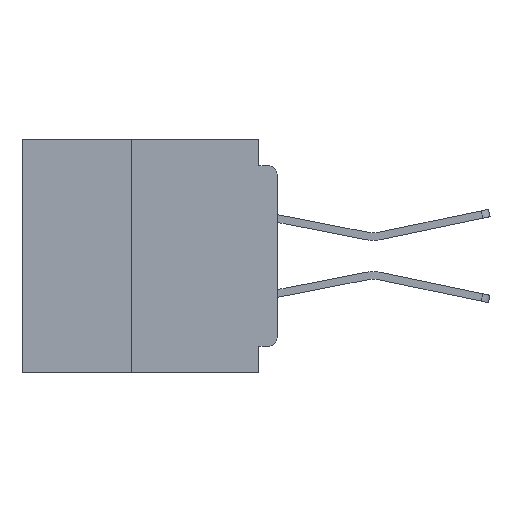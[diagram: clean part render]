
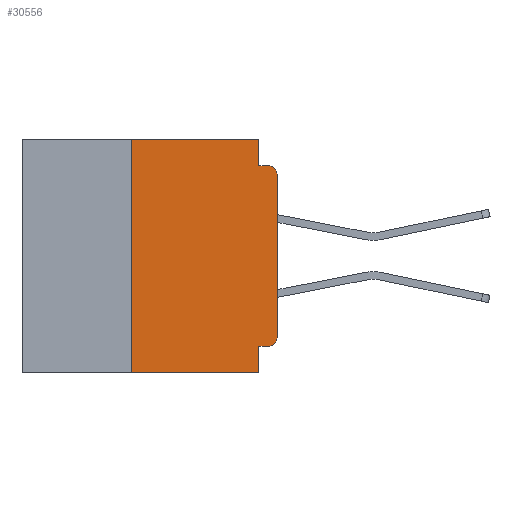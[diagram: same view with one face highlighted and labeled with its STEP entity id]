
A CAD part, left-side view. The second image highlights one B-rep face of the part: STEP entity #30556.
In plain terms, the highlighted planar face has unit normal (-1, 0, 0).
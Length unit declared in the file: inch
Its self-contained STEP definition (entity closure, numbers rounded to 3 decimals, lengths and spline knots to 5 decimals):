
#1017 = VECTOR ( 'NONE', #9681, 39.37008 ) ;
#1236 = VERTEX_POINT ( 'NONE', #1339 ) ;
#1339 = CARTESIAN_POINT ( 'NONE',  ( 0., 0.015, -0.045 ) ) ;
#1862 = ORIENTED_EDGE ( 'NONE', *, *, #42022, .F. ) ;
#1896 = ORIENTED_EDGE ( 'NONE', *, *, #35441, .F. ) ;
#3460 = VECTOR ( 'NONE', #53375, 39.37008 ) ;
#4690 = LINE ( 'NONE', #44997, #47994 ) ;
#5162 = DIRECTION ( 'NONE',  ( 0., -1., 0. ) ) ;
#5245 = VERTEX_POINT ( 'NONE', #38163 ) ;
#5361 = ORIENTED_EDGE ( 'NONE', *, *, #27050, .T. ) ;
#5423 = CARTESIAN_POINT ( 'NONE',  ( 0., 0.437, -0.4 ) ) ;
#6847 = ORIENTED_EDGE ( 'NONE', *, *, #15869, .F. ) ;
#7139 = CARTESIAN_POINT ( 'NONE',  ( 0., 0., 0. ) ) ;
#7909 = VECTOR ( 'NONE', #19508, 39.37008 ) ;
#8006 = DIRECTION ( 'NONE',  ( 1., 0., 0. ) ) ;
#8159 = VERTEX_POINT ( 'NONE', #43054 ) ;
#8168 = CIRCLE ( 'NONE', #32516, 0.015 ) ;
#8342 = ORIENTED_EDGE ( 'NONE', *, *, #15231, .T. ) ;
#9681 = DIRECTION ( 'NONE',  ( 0., -1., 0. ) ) ;
#10176 = AXIS2_PLACEMENT_3D ( 'NONE', #38931, #13913, #43147 ) ;
#11632 = DIRECTION ( 'NONE',  ( 0., -1., 0. ) ) ;
#11812 = CARTESIAN_POINT ( 'NONE',  ( 0., 0.437, 0. ) ) ;
#13487 = CARTESIAN_POINT ( 'NONE',  ( 0., 0.25, -0.4 ) ) ;
#13815 = CARTESIAN_POINT ( 'NONE',  ( 0., 0.031, -0.4 ) ) ;
#13913 = DIRECTION ( 'NONE',  ( -1., 0., 0. ) ) ;
#14528 = CARTESIAN_POINT ( 'NONE',  ( 0., 0.031, 0. ) ) ;
#14894 = VERTEX_POINT ( 'NONE', #17578 ) ;
#15231 = EDGE_CURVE ( 'NONE', #5245, #53070, #37618, .T. ) ;
#15804 = VERTEX_POINT ( 'NONE', #32014 ) ;
#15869 = EDGE_CURVE ( 'NONE', #14894, #30170, #4690, .T. ) ;
#16266 = EDGE_CURVE ( 'NONE', #15804, #14894, #40784, .T. ) ;
#17531 = VERTEX_POINT ( 'NONE', #14528 ) ;
#17578 = CARTESIAN_POINT ( 'NONE',  ( 0., 0.031, -0.355 ) ) ;
#18138 = ORIENTED_EDGE ( 'NONE', *, *, #53557, .T. ) ;
#19508 = DIRECTION ( 'NONE',  ( 0., 0., -1. ) ) ;
#21286 = FACE_OUTER_BOUND ( 'NONE', #34796, .T. ) ;
#22090 = DIRECTION ( 'NONE',  ( -1., 0., 0. ) ) ;
#22170 = VERTEX_POINT ( 'NONE', #13487 ) ;
#23447 = CARTESIAN_POINT ( 'NONE',  ( 0., 0., -0.355 ) ) ;
#23816 = VECTOR ( 'NONE', #11632, 39.37008 ) ;
#25314 = ORIENTED_EDGE ( 'NONE', *, *, #38637, .F. ) ;
#26413 = LINE ( 'NONE', #11812, #23816 ) ;
#27050 = EDGE_CURVE ( 'NONE', #22170, #30170, #34621, .T. ) ;
#28371 = DIRECTION ( 'NONE',  ( 0., 0., -1. ) ) ;
#28968 = PLANE ( 'NONE',  #41947 ) ;
#29868 = EDGE_CURVE ( 'NONE', #22170, #34425, #36995, .T. ) ;
#30170 = VERTEX_POINT ( 'NONE', #13815 ) ;
#30267 = LINE ( 'NONE', #52787, #7909 ) ;
#30556 = ADVANCED_FACE ( 'NONE', ( #21286 ), #28968, .F. ) ;
#31398 = CARTESIAN_POINT ( 'NONE',  ( 0., 0., -0.06 ) ) ;
#32014 = CARTESIAN_POINT ( 'NONE',  ( 0., 0.015, -0.355 ) ) ;
#32516 = AXIS2_PLACEMENT_3D ( 'NONE', #47049, #22090, #51180 ) ;
#32575 = CIRCLE ( 'NONE', #10176, 0.015 ) ;
#32666 = LINE ( 'NONE', #51106, #53475 ) ;
#32994 = ORIENTED_EDGE ( 'NONE', *, *, #29868, .F. ) ;
#34425 = VERTEX_POINT ( 'NONE', #48757 ) ;
#34621 = LINE ( 'NONE', #5423, #1017 ) ;
#34796 = EDGE_LOOP ( 'NONE', ( #8342, #18138, #25314, #1896, #1862, #32994, #5361, #6847, #50646, #39757 ) ) ;
#35441 = EDGE_CURVE ( 'NONE', #17531, #8159, #30267, .T. ) ;
#36465 = DIRECTION ( 'NONE',  ( 0., 0., 1. ) ) ;
#36995 = LINE ( 'NONE', #45095, #3460 ) ;
#37329 = DIRECTION ( 'NONE',  ( 0., 0., -1. ) ) ;
#37618 = LINE ( 'NONE', #7139, #48718 ) ;
#38163 = CARTESIAN_POINT ( 'NONE',  ( 0., 0., -0.34 ) ) ;
#38637 = EDGE_CURVE ( 'NONE', #8159, #1236, #32666, .T. ) ;
#38931 = CARTESIAN_POINT ( 'NONE',  ( 0., 0.015, -0.34 ) ) ;
#39757 = ORIENTED_EDGE ( 'NONE', *, *, #45279, .T. ) ;
#40784 = LINE ( 'NONE', #23447, #53091 ) ;
#41947 = AXIS2_PLACEMENT_3D ( 'NONE', #49707, #8006, #37329 ) ;
#42022 = EDGE_CURVE ( 'NONE', #34425, #17531, #26413, .T. ) ;
#43054 = CARTESIAN_POINT ( 'NONE',  ( 0., 0.031, -0.045 ) ) ;
#43147 = DIRECTION ( 'NONE',  ( 0., 0., -1. ) ) ;
#44997 = CARTESIAN_POINT ( 'NONE',  ( 0., 0.031, -0.4 ) ) ;
#45095 = CARTESIAN_POINT ( 'NONE',  ( 0., 0.25, -0.4 ) ) ;
#45279 = EDGE_CURVE ( 'NONE', #15804, #5245, #32575, .T. ) ;
#47049 = CARTESIAN_POINT ( 'NONE',  ( 0., 0.015, -0.06 ) ) ;
#47994 = VECTOR ( 'NONE', #28371, 39.37008 ) ;
#48718 = VECTOR ( 'NONE', #36465, 39.37008 ) ;
#48757 = CARTESIAN_POINT ( 'NONE',  ( 0., 0.25, 0. ) ) ;
#49707 = CARTESIAN_POINT ( 'NONE',  ( 0., 0.437, 0. ) ) ;
#50646 = ORIENTED_EDGE ( 'NONE', *, *, #16266, .F. ) ;
#51106 = CARTESIAN_POINT ( 'NONE',  ( 0., 0., -0.045 ) ) ;
#51180 = DIRECTION ( 'NONE',  ( 0., 0., -1. ) ) ;
#52533 = DIRECTION ( 'NONE',  ( 0., 1., 0. ) ) ;
#52787 = CARTESIAN_POINT ( 'NONE',  ( 0., 0.031, 0. ) ) ;
#53070 = VERTEX_POINT ( 'NONE', #31398 ) ;
#53091 = VECTOR ( 'NONE', #52533, 39.37008 ) ;
#53375 = DIRECTION ( 'NONE',  ( 0., 0., 1. ) ) ;
#53475 = VECTOR ( 'NONE', #5162, 39.37008 ) ;
#53557 = EDGE_CURVE ( 'NONE', #53070, #1236, #8168, .T. ) ;
